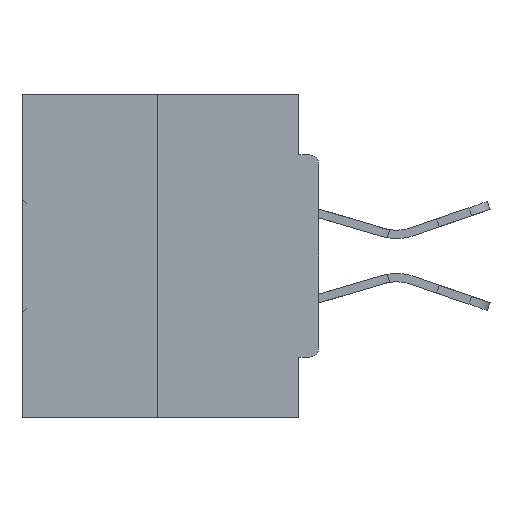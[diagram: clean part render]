
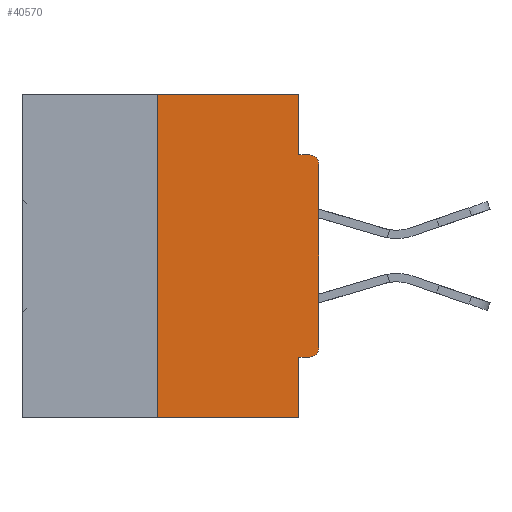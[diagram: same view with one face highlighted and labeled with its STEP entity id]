
A CAD part, left-side view. The second image highlights one B-rep face of the part: STEP entity #40570.
In plain terms, the highlighted planar face has unit normal (-1, 0, 0).
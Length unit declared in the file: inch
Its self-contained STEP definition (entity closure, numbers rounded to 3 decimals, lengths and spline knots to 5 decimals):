
#665 = VERTEX_POINT ( 'NONE', #26553 ) ;
#1022 = VERTEX_POINT ( 'NONE', #17394 ) ;
#1053 = VERTEX_POINT ( 'NONE', #37048 ) ;
#1491 = DIRECTION ( 'NONE',  ( 0., 0., 1. ) ) ;
#3492 = EDGE_CURVE ( 'NONE', #19015, #665, #8249, .T. ) ;
#4219 = ORIENTED_EDGE ( 'NONE', *, *, #6136, .T. ) ;
#4916 = VERTEX_POINT ( 'NONE', #23795 ) ;
#5418 = DIRECTION ( 'NONE',  ( 0., 0., -1. ) ) ;
#5457 = VECTOR ( 'NONE', #7784, 39.37008 ) ;
#6099 = DIRECTION ( 'NONE',  ( 0., 0., 1. ) ) ;
#6136 = EDGE_CURVE ( 'NONE', #665, #1022, #24836, .T. ) ;
#6332 = CARTESIAN_POINT ( 'NONE',  ( 0., 0., 0. ) ) ;
#6843 = CARTESIAN_POINT ( 'NONE',  ( 0., 0.015, -0.3915 ) ) ;
#6932 = PLANE ( 'NONE',  #37478 ) ;
#7784 = DIRECTION ( 'NONE',  ( 0., -1., 0. ) ) ;
#8249 = CIRCLE ( 'NONE', #11306, 0.015 ) ;
#8834 = CARTESIAN_POINT ( 'NONE',  ( 0., 0.015, -0.0935 ) ) ;
#10664 = CARTESIAN_POINT ( 'NONE',  ( 0., 0.015, -0.4065 ) ) ;
#11284 = DIRECTION ( 'NONE',  ( 0., 0., -1. ) ) ;
#11306 = AXIS2_PLACEMENT_3D ( 'NONE', #6843, #14063, #17437 ) ;
#11595 = EDGE_LOOP ( 'NONE', ( #32215, #27187, #19645, #13516, #38509, #43407, #4219, #27500, #25338, #12846 ) ) ;
#11628 = DIRECTION ( 'NONE',  ( -1., 0., 0. ) ) ;
#12726 = DIRECTION ( 'NONE',  ( 0., -1., 0. ) ) ;
#12846 = ORIENTED_EDGE ( 'NONE', *, *, #42510, .F. ) ;
#13516 = ORIENTED_EDGE ( 'NONE', *, *, #16512, .F. ) ;
#14063 = DIRECTION ( 'NONE',  ( -1., 0., 0. ) ) ;
#15449 = EDGE_CURVE ( 'NONE', #19015, #4916, #37374, .T. ) ;
#15541 = DIRECTION ( 'NONE',  ( 0., 1., 0. ) ) ;
#15989 = VERTEX_POINT ( 'NONE', #23633 ) ;
#16512 = EDGE_CURVE ( 'NONE', #4916, #18825, #22321, .T. ) ;
#16858 = LINE ( 'NONE', #27888, #23417 ) ;
#17394 = CARTESIAN_POINT ( 'NONE',  ( 0., 0., -0.1085 ) ) ;
#17420 = CARTESIAN_POINT ( 'NONE',  ( 0., 0.031, -0.5 ) ) ;
#17437 = DIRECTION ( 'NONE',  ( 0., 0., -1. ) ) ;
#18057 = VERTEX_POINT ( 'NONE', #47130 ) ;
#18825 = VERTEX_POINT ( 'NONE', #17420 ) ;
#19015 = VERTEX_POINT ( 'NONE', #10664 ) ;
#19645 = ORIENTED_EDGE ( 'NONE', *, *, #38861, .T. ) ;
#20846 = VERTEX_POINT ( 'NONE', #38666 ) ;
#21148 = CARTESIAN_POINT ( 'NONE',  ( 0., 0.46, -0.5 ) ) ;
#21577 = DIRECTION ( 'NONE',  ( 1., 0., 0. ) ) ;
#22321 = LINE ( 'NONE', #36481, #39125 ) ;
#23417 = VECTOR ( 'NONE', #1491, 39.37008 ) ;
#23633 = CARTESIAN_POINT ( 'NONE',  ( 0., 0.25, 0. ) ) ;
#23687 = LINE ( 'NONE', #38311, #41464 ) ;
#23795 = CARTESIAN_POINT ( 'NONE',  ( 0., 0.031, -0.4065 ) ) ;
#24232 = LINE ( 'NONE', #42013, #41601 ) ;
#24836 = LINE ( 'NONE', #6332, #46660 ) ;
#25004 = EDGE_CURVE ( 'NONE', #1022, #39565, #27040, .T. ) ;
#25338 = ORIENTED_EDGE ( 'NONE', *, *, #26843, .F. ) ;
#26049 = LINE ( 'NONE', #29656, #5457 ) ;
#26513 = CARTESIAN_POINT ( 'NONE',  ( 0., 0.015, -0.1085 ) ) ;
#26553 = CARTESIAN_POINT ( 'NONE',  ( 0., 0., -0.3915 ) ) ;
#26843 = EDGE_CURVE ( 'NONE', #20846, #39565, #24232, .T. ) ;
#27040 = CIRCLE ( 'NONE', #33930, 0.015 ) ;
#27187 = ORIENTED_EDGE ( 'NONE', *, *, #29509, .F. ) ;
#27500 = ORIENTED_EDGE ( 'NONE', *, *, #25004, .T. ) ;
#27888 = CARTESIAN_POINT ( 'NONE',  ( 0., 0.25, 0. ) ) ;
#28128 = LINE ( 'NONE', #21148, #45918 ) ;
#28314 = DIRECTION ( 'NONE',  ( 0., 0., -1. ) ) ;
#29509 = EDGE_CURVE ( 'NONE', #18057, #15989, #16858, .T. ) ;
#29656 = CARTESIAN_POINT ( 'NONE',  ( 0., 0.46, 0. ) ) ;
#30118 = DIRECTION ( 'NONE',  ( 0., 0., -1. ) ) ;
#31924 = FACE_OUTER_BOUND ( 'NONE', #11595, .T. ) ;
#32215 = ORIENTED_EDGE ( 'NONE', *, *, #44887, .F. ) ;
#33544 = CARTESIAN_POINT ( 'NONE',  ( 0., 0., -0.4065 ) ) ;
#33930 = AXIS2_PLACEMENT_3D ( 'NONE', #26513, #11628, #30118 ) ;
#36481 = CARTESIAN_POINT ( 'NONE',  ( 0., 0.031, -0.5 ) ) ;
#37048 = CARTESIAN_POINT ( 'NONE',  ( 0., 0.031, 0. ) ) ;
#37374 = LINE ( 'NONE', #33544, #38285 ) ;
#37478 = AXIS2_PLACEMENT_3D ( 'NONE', #39355, #21577, #28314 ) ;
#38285 = VECTOR ( 'NONE', #15541, 39.37008 ) ;
#38311 = CARTESIAN_POINT ( 'NONE',  ( 0., 0.031, 0. ) ) ;
#38509 = ORIENTED_EDGE ( 'NONE', *, *, #15449, .F. ) ;
#38666 = CARTESIAN_POINT ( 'NONE',  ( 0., 0.031, -0.0935 ) ) ;
#38861 = EDGE_CURVE ( 'NONE', #18057, #18825, #28128, .T. ) ;
#39125 = VECTOR ( 'NONE', #11284, 39.37008 ) ;
#39355 = CARTESIAN_POINT ( 'NONE',  ( 0., 0.46, 0. ) ) ;
#39565 = VERTEX_POINT ( 'NONE', #8834 ) ;
#40570 = ADVANCED_FACE ( 'NONE', ( #31924 ), #6932, .F. ) ;
#41464 = VECTOR ( 'NONE', #5418, 39.37008 ) ;
#41601 = VECTOR ( 'NONE', #12726, 39.37008 ) ;
#42013 = CARTESIAN_POINT ( 'NONE',  ( 0., 0., -0.0935 ) ) ;
#42510 = EDGE_CURVE ( 'NONE', #1053, #20846, #23687, .T. ) ;
#43407 = ORIENTED_EDGE ( 'NONE', *, *, #3492, .T. ) ;
#44887 = EDGE_CURVE ( 'NONE', #15989, #1053, #26049, .T. ) ;
#45918 = VECTOR ( 'NONE', #46640, 39.37008 ) ;
#46640 = DIRECTION ( 'NONE',  ( 0., -1., 0. ) ) ;
#46660 = VECTOR ( 'NONE', #6099, 39.37008 ) ;
#47130 = CARTESIAN_POINT ( 'NONE',  ( 0., 0.25, -0.5 ) ) ;
